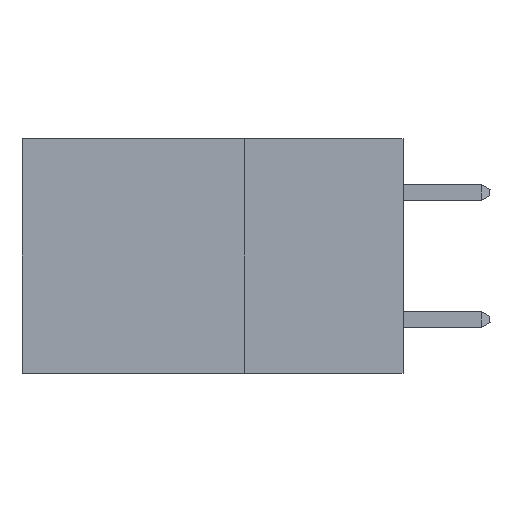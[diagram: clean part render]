
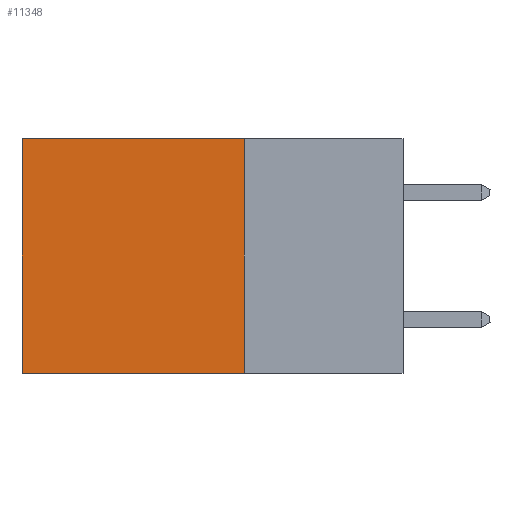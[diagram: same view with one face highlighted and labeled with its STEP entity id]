
A CAD part, left-side view. The second image highlights one B-rep face of the part: STEP entity #11348.
In plain terms, the highlighted planar face has unit normal (-1, 0, 0).
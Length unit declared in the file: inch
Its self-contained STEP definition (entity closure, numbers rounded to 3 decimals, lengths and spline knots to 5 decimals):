
#255 = VECTOR ( 'NONE', #10076, 39.37008 ) ;
#1499 = LINE ( 'NONE', #23128, #16970 ) ;
#3304 = VERTEX_POINT ( 'NONE', #7536 ) ;
#3692 = DIRECTION ( 'NONE',  ( 0., 0., -1. ) ) ;
#3868 = CARTESIAN_POINT ( 'NONE',  ( 0.2875, 0.6, -0.37 ) ) ;
#5267 = EDGE_CURVE ( 'NONE', #21122, #5681, #1499, .T. ) ;
#5418 = ORIENTED_EDGE ( 'NONE', *, *, #18359, .F. ) ;
#5489 = CARTESIAN_POINT ( 'NONE',  ( 0.2875, 0.25, 0. ) ) ;
#5681 = VERTEX_POINT ( 'NONE', #3868 ) ;
#7536 = CARTESIAN_POINT ( 'NONE',  ( 0.2875, 0.25, -0.37 ) ) ;
#7788 = VECTOR ( 'NONE', #26444, 39.37008 ) ;
#8172 = ORIENTED_EDGE ( 'NONE', *, *, #15012, .F. ) ;
#8518 = DIRECTION ( 'NONE',  ( 0., 1., 0. ) ) ;
#9300 = FACE_OUTER_BOUND ( 'NONE', #10963, .T. ) ;
#9674 = ORIENTED_EDGE ( 'NONE', *, *, #5267, .T. ) ;
#10076 = DIRECTION ( 'NONE',  ( 0., 1., 0. ) ) ;
#10963 = EDGE_LOOP ( 'NONE', ( #9674, #5418, #8172, #13550 ) ) ;
#10990 = CARTESIAN_POINT ( 'NONE',  ( 0.2875, 0.25, 0. ) ) ;
#11016 = VERTEX_POINT ( 'NONE', #10990 ) ;
#11348 = ADVANCED_FACE ( 'NONE', ( #9300 ), #12068, .F. ) ;
#12068 = PLANE ( 'NONE',  #20505 ) ;
#13550 = ORIENTED_EDGE ( 'NONE', *, *, #13752, .T. ) ;
#13752 = EDGE_CURVE ( 'NONE', #11016, #21122, #17073, .T. ) ;
#15012 = EDGE_CURVE ( 'NONE', #11016, #3304, #18969, .T. ) ;
#15120 = VECTOR ( 'NONE', #8518, 39.37008 ) ;
#16295 = DIRECTION ( 'NONE',  ( 1., 0., 0. ) ) ;
#16970 = VECTOR ( 'NONE', #21042, 39.37008 ) ;
#17073 = LINE ( 'NONE', #26701, #255 ) ;
#18359 = EDGE_CURVE ( 'NONE', #3304, #5681, #20718, .T. ) ;
#18969 = LINE ( 'NONE', #5489, #7788 ) ;
#20041 = CARTESIAN_POINT ( 'NONE',  ( 0.2875, 0.6, 0. ) ) ;
#20505 = AXIS2_PLACEMENT_3D ( 'NONE', #26667, #16295, #3692 ) ;
#20718 = LINE ( 'NONE', #23170, #15120 ) ;
#21042 = DIRECTION ( 'NONE',  ( 0., 0., -1. ) ) ;
#21122 = VERTEX_POINT ( 'NONE', #20041 ) ;
#23128 = CARTESIAN_POINT ( 'NONE',  ( 0.2875, 0.6, 0. ) ) ;
#23170 = CARTESIAN_POINT ( 'NONE',  ( 0.2875, 0.25, -0.37 ) ) ;
#26444 = DIRECTION ( 'NONE',  ( 0., 0., -1. ) ) ;
#26667 = CARTESIAN_POINT ( 'NONE',  ( 0.2875, 0.25, 0. ) ) ;
#26701 = CARTESIAN_POINT ( 'NONE',  ( 0.2875, 0.25, 0. ) ) ;
